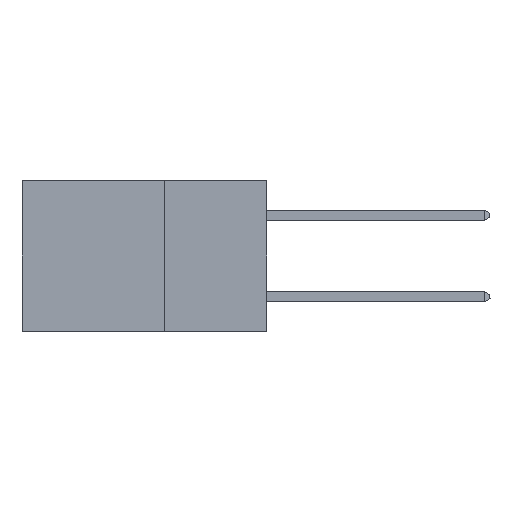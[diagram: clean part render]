
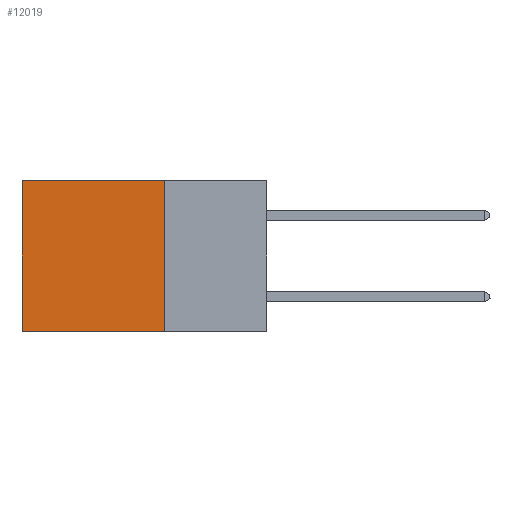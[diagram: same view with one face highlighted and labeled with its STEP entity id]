
A CAD part, left-side view. The second image highlights one B-rep face of the part: STEP entity #12019.
In plain terms, the highlighted planar face has unit normal (-1, 0, 0).
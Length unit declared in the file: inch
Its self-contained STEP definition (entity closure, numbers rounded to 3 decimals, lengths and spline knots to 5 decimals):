
#630 = EDGE_LOOP ( 'NONE', ( #982, #7384, #5336, #3962 ) ) ;
#857 = FACE_OUTER_BOUND ( 'NONE', #630, .T. ) ;
#982 = ORIENTED_EDGE ( 'NONE', *, *, #10796, .T. ) ;
#1178 = VECTOR ( 'NONE', #2216, 39.37008 ) ;
#2216 = DIRECTION ( 'NONE',  ( 0., 0., -1. ) ) ;
#2307 = CARTESIAN_POINT ( 'NONE',  ( 0.2875, 0.25, 0. ) ) ;
#2309 = CARTESIAN_POINT ( 'NONE',  ( 0.2875, 0.6, -0.37 ) ) ;
#2532 = VERTEX_POINT ( 'NONE', #5921 ) ;
#2808 = VERTEX_POINT ( 'NONE', #2309 ) ;
#3328 = VECTOR ( 'NONE', #4449, 39.37008 ) ;
#3515 = VECTOR ( 'NONE', #8484, 39.37008 ) ;
#3884 = VECTOR ( 'NONE', #11950, 39.37008 ) ;
#3962 = ORIENTED_EDGE ( 'NONE', *, *, #12739, .T. ) ;
#4449 = DIRECTION ( 'NONE',  ( 0., 0., -1. ) ) ;
#4605 = DIRECTION ( 'NONE',  ( 0., 0., -1. ) ) ;
#4953 = CARTESIAN_POINT ( 'NONE',  ( 0.2875, 0.25, -0.37 ) ) ;
#5140 = EDGE_CURVE ( 'NONE', #7850, #2532, #9545, .T. ) ;
#5336 = ORIENTED_EDGE ( 'NONE', *, *, #5140, .F. ) ;
#5921 = CARTESIAN_POINT ( 'NONE',  ( 0.2875, 0.25, -0.37 ) ) ;
#6312 = LINE ( 'NONE', #4953, #3884 ) ;
#6621 = LINE ( 'NONE', #13301, #3515 ) ;
#6714 = CARTESIAN_POINT ( 'NONE',  ( 0.2875, 0.6, 0. ) ) ;
#7384 = ORIENTED_EDGE ( 'NONE', *, *, #9288, .F. ) ;
#7850 = VERTEX_POINT ( 'NONE', #2307 ) ;
#8484 = DIRECTION ( 'NONE',  ( 0., 1., 0. ) ) ;
#8698 = PLANE ( 'NONE',  #11625 ) ;
#8848 = LINE ( 'NONE', #6714, #3328 ) ;
#9288 = EDGE_CURVE ( 'NONE', #2532, #2808, #6312, .T. ) ;
#9545 = LINE ( 'NONE', #12323, #1178 ) ;
#9685 = CARTESIAN_POINT ( 'NONE',  ( 0.2875, 0.25, 0. ) ) ;
#10372 = CARTESIAN_POINT ( 'NONE',  ( 0.2875, 0.6, 0. ) ) ;
#10662 = DIRECTION ( 'NONE',  ( 1., 0., 0. ) ) ;
#10796 = EDGE_CURVE ( 'NONE', #12684, #2808, #8848, .T. ) ;
#11625 = AXIS2_PLACEMENT_3D ( 'NONE', #9685, #10662, #4605 ) ;
#11950 = DIRECTION ( 'NONE',  ( 0., 1., 0. ) ) ;
#12019 = ADVANCED_FACE ( 'NONE', ( #857 ), #8698, .F. ) ;
#12323 = CARTESIAN_POINT ( 'NONE',  ( 0.2875, 0.25, 0. ) ) ;
#12684 = VERTEX_POINT ( 'NONE', #10372 ) ;
#12739 = EDGE_CURVE ( 'NONE', #7850, #12684, #6621, .T. ) ;
#13301 = CARTESIAN_POINT ( 'NONE',  ( 0.2875, 0.25, 0. ) ) ;
